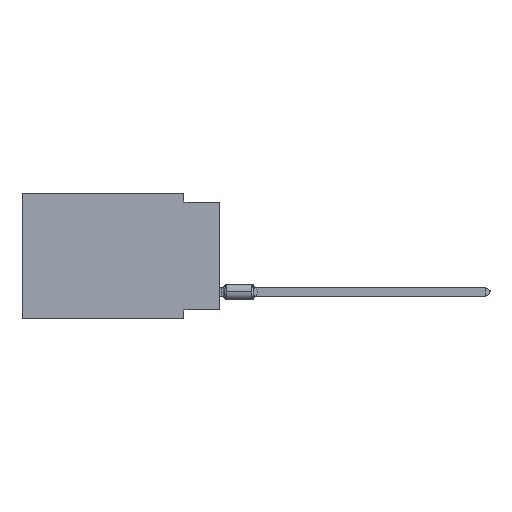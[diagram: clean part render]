
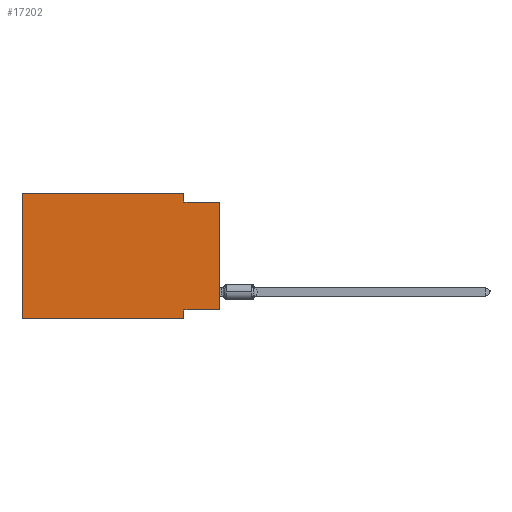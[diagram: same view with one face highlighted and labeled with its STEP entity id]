
A CAD part, left-side view. The second image highlights one B-rep face of the part: STEP entity #17202.
In plain terms, the highlighted planar face has unit normal (-1, 0, 0).
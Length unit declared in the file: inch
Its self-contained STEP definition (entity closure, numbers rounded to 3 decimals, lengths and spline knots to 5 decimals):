
#429 = DIRECTION ( 'NONE',  ( 0., 0., 1. ) ) ;
#1039 = LINE ( 'NONE', #6775, #19258 ) ;
#2634 = LINE ( 'NONE', #41379, #13895 ) ;
#3500 = DIRECTION ( 'NONE',  ( 1., 0., 0. ) ) ;
#4645 = VERTEX_POINT ( 'NONE', #4830 ) ;
#4830 = CARTESIAN_POINT ( 'NONE',  ( 0., 0.1, -0.025 ) ) ;
#6682 = DIRECTION ( 'NONE',  ( 0., 1., 0. ) ) ;
#6775 = CARTESIAN_POINT ( 'NONE',  ( 0., 0.1, 0. ) ) ;
#6837 = CARTESIAN_POINT ( 'NONE',  ( 0., 0., -0.325 ) ) ;
#7983 = CARTESIAN_POINT ( 'NONE',  ( 0., 0.55, 0. ) ) ;
#8987 = ORIENTED_EDGE ( 'NONE', *, *, #25419, .T. ) ;
#11075 = VERTEX_POINT ( 'NONE', #6837 ) ;
#13832 = LINE ( 'NONE', #43304, #33368 ) ;
#13895 = VECTOR ( 'NONE', #36249, 39.37008 ) ;
#15647 = CARTESIAN_POINT ( 'NONE',  ( 0., 0., -0.325 ) ) ;
#15889 = EDGE_CURVE ( 'NONE', #4645, #40640, #26216, .T. ) ;
#16649 = EDGE_CURVE ( 'NONE', #42255, #4645, #1039, .T. ) ;
#17202 = ADVANCED_FACE ( 'NONE', ( #23024 ), #57257, .F. ) ;
#18896 = CARTESIAN_POINT ( 'NONE',  ( 0., 0.55, -0.35 ) ) ;
#18956 = DIRECTION ( 'NONE',  ( 0., -1., 0. ) ) ;
#19258 = VECTOR ( 'NONE', #46145, 39.37008 ) ;
#19313 = LINE ( 'NONE', #29251, #39025 ) ;
#19377 = CARTESIAN_POINT ( 'NONE',  ( 0., 0., -0.025 ) ) ;
#20143 = LINE ( 'NONE', #15647, #42886 ) ;
#20334 = CARTESIAN_POINT ( 'NONE',  ( 0., 0.1, -0.325 ) ) ;
#20474 = CARTESIAN_POINT ( 'NONE',  ( 0., 0., -0.025 ) ) ;
#21167 = VECTOR ( 'NONE', #40629, 39.37008 ) ;
#23024 = FACE_OUTER_BOUND ( 'NONE', #50891, .T. ) ;
#23994 = DIRECTION ( 'NONE',  ( 0., 0., -1. ) ) ;
#25357 = DIRECTION ( 'NONE',  ( 0., 0., 1. ) ) ;
#25419 = EDGE_CURVE ( 'NONE', #11075, #40640, #35580, .T. ) ;
#25510 = ORIENTED_EDGE ( 'NONE', *, *, #50150, .F. ) ;
#26216 = LINE ( 'NONE', #20474, #21167 ) ;
#27828 = DIRECTION ( 'NONE',  ( 0., 0., -1. ) ) ;
#29251 = CARTESIAN_POINT ( 'NONE',  ( 0., 0.55, 0. ) ) ;
#32202 = VERTEX_POINT ( 'NONE', #50810 ) ;
#33283 = LINE ( 'NONE', #47381, #51746 ) ;
#33368 = VECTOR ( 'NONE', #18956, 39.37008 ) ;
#34342 = CARTESIAN_POINT ( 'NONE',  ( 0., 0., 0. ) ) ;
#34388 = ORIENTED_EDGE ( 'NONE', *, *, #54497, .F. ) ;
#35580 = LINE ( 'NONE', #34342, #43274 ) ;
#35754 = EDGE_CURVE ( 'NONE', #42533, #42255, #2634, .T. ) ;
#36249 = DIRECTION ( 'NONE',  ( 0., -1., 0. ) ) ;
#36525 = ORIENTED_EDGE ( 'NONE', *, *, #61816, .F. ) ;
#36876 = CARTESIAN_POINT ( 'NONE',  ( 0., 0.55, 0. ) ) ;
#36995 = ORIENTED_EDGE ( 'NONE', *, *, #15889, .F. ) ;
#38817 = VERTEX_POINT ( 'NONE', #18896 ) ;
#39025 = VECTOR ( 'NONE', #429, 39.37008 ) ;
#40629 = DIRECTION ( 'NONE',  ( 0., -1., 0. ) ) ;
#40640 = VERTEX_POINT ( 'NONE', #19377 ) ;
#41379 = CARTESIAN_POINT ( 'NONE',  ( 0., 0.55, 0. ) ) ;
#42255 = VERTEX_POINT ( 'NONE', #63144 ) ;
#42533 = VERTEX_POINT ( 'NONE', #36876 ) ;
#42886 = VECTOR ( 'NONE', #6682, 39.37008 ) ;
#43274 = VECTOR ( 'NONE', #25357, 39.37008 ) ;
#43304 = CARTESIAN_POINT ( 'NONE',  ( 0., 0.55, -0.35 ) ) ;
#43447 = ORIENTED_EDGE ( 'NONE', *, *, #35754, .F. ) ;
#45190 = EDGE_CURVE ( 'NONE', #38817, #32202, #13832, .T. ) ;
#45470 = ORIENTED_EDGE ( 'NONE', *, *, #45190, .T. ) ;
#46145 = DIRECTION ( 'NONE',  ( 0., 0., -1. ) ) ;
#46165 = ORIENTED_EDGE ( 'NONE', *, *, #16649, .F. ) ;
#47381 = CARTESIAN_POINT ( 'NONE',  ( 0., 0.1, -0.35 ) ) ;
#48934 = AXIS2_PLACEMENT_3D ( 'NONE', #7983, #3500, #27828 ) ;
#50150 = EDGE_CURVE ( 'NONE', #11075, #58084, #20143, .T. ) ;
#50810 = CARTESIAN_POINT ( 'NONE',  ( 0., 0.1, -0.35 ) ) ;
#50891 = EDGE_LOOP ( 'NONE', ( #8987, #36995, #46165, #43447, #34388, #45470, #36525, #25510 ) ) ;
#51746 = VECTOR ( 'NONE', #23994, 39.37008 ) ;
#54497 = EDGE_CURVE ( 'NONE', #38817, #42533, #19313, .T. ) ;
#57257 = PLANE ( 'NONE',  #48934 ) ;
#58084 = VERTEX_POINT ( 'NONE', #20334 ) ;
#61816 = EDGE_CURVE ( 'NONE', #58084, #32202, #33283, .T. ) ;
#63144 = CARTESIAN_POINT ( 'NONE',  ( 0., 0.1, 0. ) ) ;
